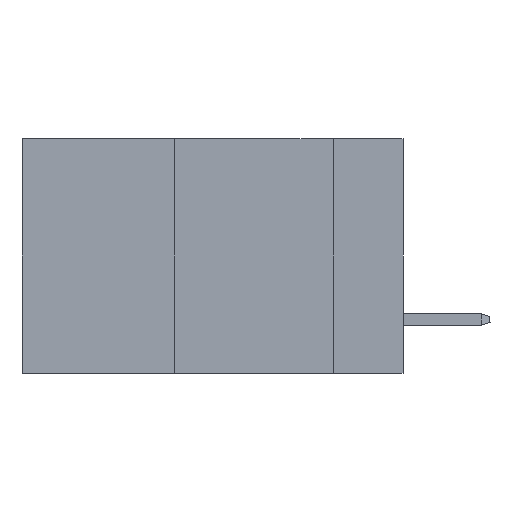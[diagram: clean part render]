
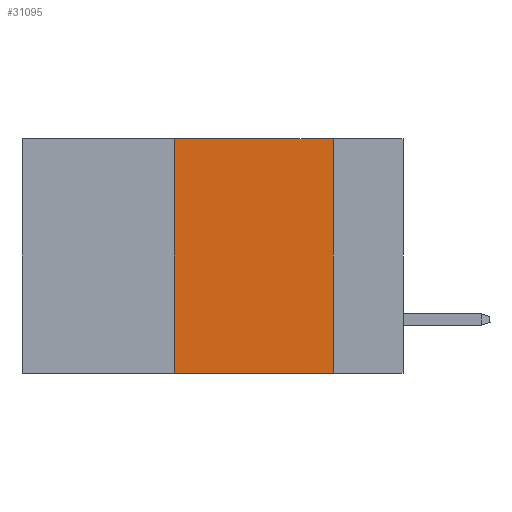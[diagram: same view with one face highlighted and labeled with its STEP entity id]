
A CAD part, left-side view. The second image highlights one B-rep face of the part: STEP entity #31095.
In plain terms, the highlighted planar face has unit normal (-1, 0, 0).
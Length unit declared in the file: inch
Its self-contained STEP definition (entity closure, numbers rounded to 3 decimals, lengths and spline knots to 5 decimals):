
#334 = LINE ( 'NONE', #32405, #16659 ) ;
#2743 = LINE ( 'NONE', #21287, #7357 ) ;
#2923 = EDGE_CURVE ( 'NONE', #7437, #28041, #334, .T. ) ;
#3090 = DIRECTION ( 'NONE',  ( 0., 0., 1. ) ) ;
#4174 = VERTEX_POINT ( 'NONE', #25947 ) ;
#5466 = AXIS2_PLACEMENT_3D ( 'NONE', #31852, #15529, #18629 ) ;
#7257 = ORIENTED_EDGE ( 'NONE', *, *, #25418, .F. ) ;
#7290 = LINE ( 'NONE', #25692, #13122 ) ;
#7357 = VECTOR ( 'NONE', #3090, 39.37008 ) ;
#7437 = VERTEX_POINT ( 'NONE', #12730 ) ;
#7566 = PLANE ( 'NONE',  #5466 ) ;
#8108 = DIRECTION ( 'NONE',  ( 0., 0., -1. ) ) ;
#8975 = VERTEX_POINT ( 'NONE', #23390 ) ;
#9469 = CARTESIAN_POINT ( 'NONE',  ( 0., 0.6, 0. ) ) ;
#12450 = ORIENTED_EDGE ( 'NONE', *, *, #31873, .F. ) ;
#12730 = CARTESIAN_POINT ( 'NONE',  ( 0., 0.11, 0. ) ) ;
#12840 = DIRECTION ( 'NONE',  ( 0., -1., 0. ) ) ;
#13122 = VECTOR ( 'NONE', #12840, 39.37008 ) ;
#15529 = DIRECTION ( 'NONE',  ( 1., 0., 0. ) ) ;
#16659 = VECTOR ( 'NONE', #8108, 39.37008 ) ;
#17412 = LINE ( 'NONE', #9469, #33487 ) ;
#18629 = DIRECTION ( 'NONE',  ( 0., 0., -1. ) ) ;
#19941 = CARTESIAN_POINT ( 'NONE',  ( 0., 0.11, -0.37 ) ) ;
#21287 = CARTESIAN_POINT ( 'NONE',  ( 0., 0.36, 0. ) ) ;
#23390 = CARTESIAN_POINT ( 'NONE',  ( 0., 0.36, 0. ) ) ;
#25418 = EDGE_CURVE ( 'NONE', #8975, #7437, #17412, .T. ) ;
#25692 = CARTESIAN_POINT ( 'NONE',  ( 0., 0.6, -0.37 ) ) ;
#25947 = CARTESIAN_POINT ( 'NONE',  ( 0., 0.36, -0.37 ) ) ;
#25982 = EDGE_LOOP ( 'NONE', ( #30525, #7257, #12450, #26931 ) ) ;
#26931 = ORIENTED_EDGE ( 'NONE', *, *, #28051, .T. ) ;
#28041 = VERTEX_POINT ( 'NONE', #19941 ) ;
#28051 = EDGE_CURVE ( 'NONE', #4174, #28041, #7290, .T. ) ;
#30525 = ORIENTED_EDGE ( 'NONE', *, *, #2923, .F. ) ;
#30823 = DIRECTION ( 'NONE',  ( 0., -1., 0. ) ) ;
#31095 = ADVANCED_FACE ( 'NONE', ( #33918 ), #7566, .F. ) ;
#31852 = CARTESIAN_POINT ( 'NONE',  ( 0., 0.6, 0. ) ) ;
#31873 = EDGE_CURVE ( 'NONE', #4174, #8975, #2743, .T. ) ;
#32405 = CARTESIAN_POINT ( 'NONE',  ( 0., 0.11, 0. ) ) ;
#33487 = VECTOR ( 'NONE', #30823, 39.37008 ) ;
#33918 = FACE_OUTER_BOUND ( 'NONE', #25982, .T. ) ;
